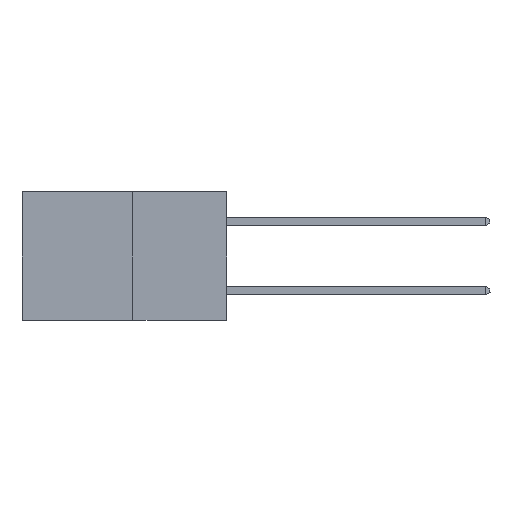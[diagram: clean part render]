
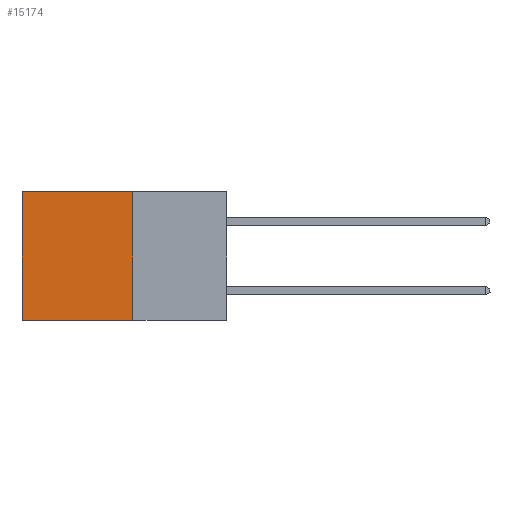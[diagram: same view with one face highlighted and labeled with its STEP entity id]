
A CAD part, left-side view. The second image highlights one B-rep face of the part: STEP entity #15174.
In plain terms, the highlighted planar face has unit normal (-1, 0, 0).
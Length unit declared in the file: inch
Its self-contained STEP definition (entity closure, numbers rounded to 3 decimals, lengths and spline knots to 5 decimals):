
#334 = EDGE_CURVE ( 'NONE', #13974, #11455, #16324, .T. ) ;
#1107 = DIRECTION ( 'NONE',  ( 0., 1., 0. ) ) ;
#1740 = VECTOR ( 'NONE', #1107, 39.37008 ) ;
#2179 = PLANE ( 'NONE',  #9895 ) ;
#2784 = EDGE_CURVE ( 'NONE', #8628, #11455, #8726, .T. ) ;
#3649 = DIRECTION ( 'NONE',  ( 0., 0., -1. ) ) ;
#3794 = CARTESIAN_POINT ( 'NONE',  ( 0.277, 0.59, -0.37 ) ) ;
#3935 = DIRECTION ( 'NONE',  ( 1., 0., 0. ) ) ;
#4228 = CARTESIAN_POINT ( 'NONE',  ( 0.277, 0.27, 0. ) ) ;
#5798 = VERTEX_POINT ( 'NONE', #4228 ) ;
#6193 = CARTESIAN_POINT ( 'NONE',  ( 0.277, 0.59, -0.37 ) ) ;
#6819 = CARTESIAN_POINT ( 'NONE',  ( 0.277, 0.27, -0.37 ) ) ;
#6883 = DIRECTION ( 'NONE',  ( 0., 0., -1. ) ) ;
#6901 = VECTOR ( 'NONE', #6883, 39.37008 ) ;
#7480 = EDGE_CURVE ( 'NONE', #5798, #8628, #20375, .T. ) ;
#8172 = VECTOR ( 'NONE', #12343, 39.37008 ) ;
#8628 = VERTEX_POINT ( 'NONE', #13715 ) ;
#8726 = LINE ( 'NONE', #22658, #8172 ) ;
#9371 = EDGE_LOOP ( 'NONE', ( #15671, #21964, #18475, #10726 ) ) ;
#9895 = AXIS2_PLACEMENT_3D ( 'NONE', #19755, #3935, #16339 ) ;
#10726 = ORIENTED_EDGE ( 'NONE', *, *, #14790, .T. ) ;
#11455 = VERTEX_POINT ( 'NONE', #6193 ) ;
#11604 = VECTOR ( 'NONE', #3649, 39.37008 ) ;
#12343 = DIRECTION ( 'NONE',  ( 0., 1., 0. ) ) ;
#12918 = CARTESIAN_POINT ( 'NONE',  ( 0.277, 0.59, 0. ) ) ;
#13715 = CARTESIAN_POINT ( 'NONE',  ( 0.277, 0.27, -0.37 ) ) ;
#13974 = VERTEX_POINT ( 'NONE', #12918 ) ;
#14790 = EDGE_CURVE ( 'NONE', #5798, #13974, #20504, .T. ) ;
#15174 = ADVANCED_FACE ( 'NONE', ( #16398 ), #2179, .F. ) ;
#15671 = ORIENTED_EDGE ( 'NONE', *, *, #334, .T. ) ;
#16324 = LINE ( 'NONE', #3794, #11604 ) ;
#16339 = DIRECTION ( 'NONE',  ( 0., 0., -1. ) ) ;
#16398 = FACE_OUTER_BOUND ( 'NONE', #9371, .T. ) ;
#18475 = ORIENTED_EDGE ( 'NONE', *, *, #7480, .F. ) ;
#19755 = CARTESIAN_POINT ( 'NONE',  ( 0.277, 0.27, -0.37 ) ) ;
#20375 = LINE ( 'NONE', #6819, #6901 ) ;
#20504 = LINE ( 'NONE', #22203, #1740 ) ;
#21964 = ORIENTED_EDGE ( 'NONE', *, *, #2784, .F. ) ;
#22203 = CARTESIAN_POINT ( 'NONE',  ( 0.277, 0.27, 0. ) ) ;
#22658 = CARTESIAN_POINT ( 'NONE',  ( 0.277, 0.27, -0.37 ) ) ;
